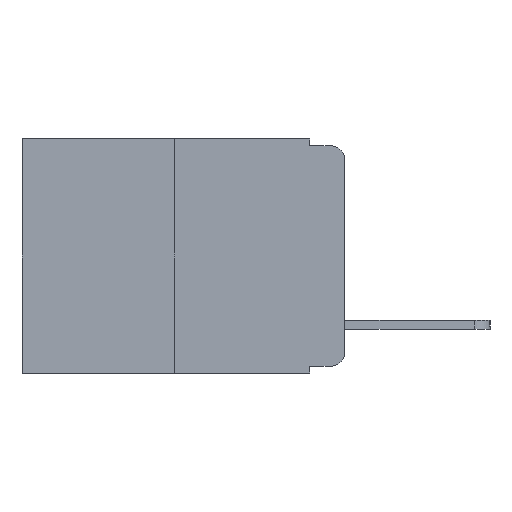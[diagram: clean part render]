
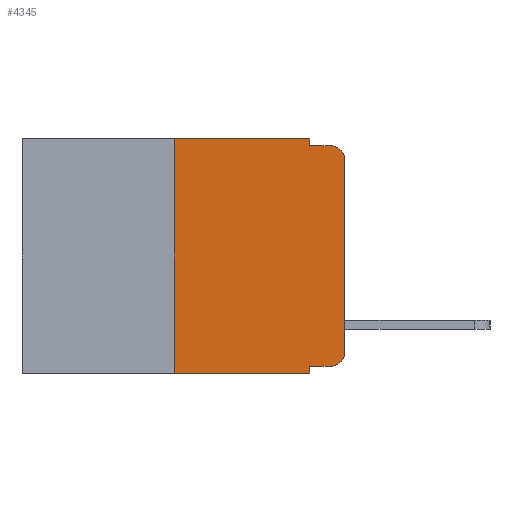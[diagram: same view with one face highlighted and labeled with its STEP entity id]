
A CAD part, left-side view. The second image highlights one B-rep face of the part: STEP entity #4345.
In plain terms, the highlighted planar face has unit normal (-1, 0, 0).
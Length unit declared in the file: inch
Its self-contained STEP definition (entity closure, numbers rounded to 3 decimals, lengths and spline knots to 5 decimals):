
#116 = VECTOR ( 'NONE', #1831, 39.37008 ) ;
#326 = CARTESIAN_POINT ( 'NONE',  ( 0., 0.051, -0.01 ) ) ;
#350 = CARTESIAN_POINT ( 'NONE',  ( 0., 0.02, -0.333 ) ) ;
#573 = VECTOR ( 'NONE', #5670, 39.37008 ) ;
#864 = CARTESIAN_POINT ( 'NONE',  ( 0., 0.473, 0. ) ) ;
#995 = EDGE_CURVE ( 'NONE', #1501, #5883, #3281, .T. ) ;
#1110 = DIRECTION ( 'NONE',  ( 0., -1., 0. ) ) ;
#1421 = VECTOR ( 'NONE', #14929, 39.37008 ) ;
#1501 = VERTEX_POINT ( 'NONE', #6995 ) ;
#1635 = ORIENTED_EDGE ( 'NONE', *, *, #4599, .F. ) ;
#1831 = DIRECTION ( 'NONE',  ( 0., 0., -1. ) ) ;
#1988 = CARTESIAN_POINT ( 'NONE',  ( 0., 0.25, 0. ) ) ;
#2081 = VERTEX_POINT ( 'NONE', #3625 ) ;
#2316 = CARTESIAN_POINT ( 'NONE',  ( 0., 0., -0.03 ) ) ;
#2392 = ORIENTED_EDGE ( 'NONE', *, *, #6445, .T. ) ;
#2616 = EDGE_CURVE ( 'NONE', #2081, #14643, #9075, .T. ) ;
#2891 = VERTEX_POINT ( 'NONE', #350 ) ;
#3139 = VECTOR ( 'NONE', #1110, 39.37008 ) ;
#3272 = LINE ( 'NONE', #5711, #3139 ) ;
#3277 = ORIENTED_EDGE ( 'NONE', *, *, #10185, .T. ) ;
#3281 = LINE ( 'NONE', #8940, #116 ) ;
#3625 = CARTESIAN_POINT ( 'NONE',  ( 0., 0.25, -0.343 ) ) ;
#3652 = AXIS2_PLACEMENT_3D ( 'NONE', #864, #13709, #5677 ) ;
#3986 = LINE ( 'NONE', #4136, #4137 ) ;
#4032 = AXIS2_PLACEMENT_3D ( 'NONE', #4738, #6208, #10890 ) ;
#4136 = CARTESIAN_POINT ( 'NONE',  ( 0., 0., 0. ) ) ;
#4137 = VECTOR ( 'NONE', #8644, 39.37008 ) ;
#4330 = ORIENTED_EDGE ( 'NONE', *, *, #12147, .T. ) ;
#4345 = ADVANCED_FACE ( 'NONE', ( #10354 ), #8130, .F. ) ;
#4388 = VERTEX_POINT ( 'NONE', #2316 ) ;
#4534 = VERTEX_POINT ( 'NONE', #11908 ) ;
#4599 = EDGE_CURVE ( 'NONE', #5883, #5077, #11755, .T. ) ;
#4738 = CARTESIAN_POINT ( 'NONE',  ( 0., 0.02, -0.313 ) ) ;
#4932 = CARTESIAN_POINT ( 'NONE',  ( 0., 0.02, -0.03 ) ) ;
#5077 = VERTEX_POINT ( 'NONE', #9718 ) ;
#5256 = CARTESIAN_POINT ( 'NONE',  ( 0., 0.473, 0. ) ) ;
#5670 = DIRECTION ( 'NONE',  ( 0., -1., 0. ) ) ;
#5677 = DIRECTION ( 'NONE',  ( 0., 0., -1. ) ) ;
#5711 = CARTESIAN_POINT ( 'NONE',  ( 0., 0.473, -0.343 ) ) ;
#5883 = VERTEX_POINT ( 'NONE', #6004 ) ;
#5895 = CARTESIAN_POINT ( 'NONE',  ( 0., 0.051, -0.333 ) ) ;
#5909 = CARTESIAN_POINT ( 'NONE',  ( 0., 0.051, -0.343 ) ) ;
#6004 = CARTESIAN_POINT ( 'NONE',  ( 0., 0.051, -0.01 ) ) ;
#6208 = DIRECTION ( 'NONE',  ( -1., 0., 0. ) ) ;
#6445 = EDGE_CURVE ( 'NONE', #4534, #4388, #3986, .T. ) ;
#6995 = CARTESIAN_POINT ( 'NONE',  ( 0., 0.051, 0. ) ) ;
#7309 = DIRECTION ( 'NONE',  ( -1., 0., 0. ) ) ;
#7410 = DIRECTION ( 'NONE',  ( 0., -1., 0. ) ) ;
#7966 = EDGE_LOOP ( 'NONE', ( #2392, #4330, #1635, #10959, #11152, #10036, #12329, #13815, #12493, #3277 ) ) ;
#8130 = PLANE ( 'NONE',  #3652 ) ;
#8278 = DIRECTION ( 'NONE',  ( 0., -1., 0. ) ) ;
#8307 = DIRECTION ( 'NONE',  ( 0., 0., -1. ) ) ;
#8644 = DIRECTION ( 'NONE',  ( 0., 0., 1. ) ) ;
#8940 = CARTESIAN_POINT ( 'NONE',  ( 0., 0.051, 0. ) ) ;
#9075 = LINE ( 'NONE', #14852, #1421 ) ;
#9117 = LINE ( 'NONE', #9195, #573 ) ;
#9195 = CARTESIAN_POINT ( 'NONE',  ( 0., 0.051, -0.333 ) ) ;
#9718 = CARTESIAN_POINT ( 'NONE',  ( 0., 0.02, -0.01 ) ) ;
#10036 = ORIENTED_EDGE ( 'NONE', *, *, #2616, .F. ) ;
#10185 = EDGE_CURVE ( 'NONE', #2891, #4534, #11129, .T. ) ;
#10354 = FACE_OUTER_BOUND ( 'NONE', #7966, .T. ) ;
#10542 = DIRECTION ( 'NONE',  ( 0., 0., -1. ) ) ;
#10698 = CARTESIAN_POINT ( 'NONE',  ( 0., 0.051, 0. ) ) ;
#10890 = DIRECTION ( 'NONE',  ( 0., 0., -1. ) ) ;
#10959 = ORIENTED_EDGE ( 'NONE', *, *, #995, .F. ) ;
#11019 = VECTOR ( 'NONE', #8278, 39.37008 ) ;
#11129 = CIRCLE ( 'NONE', #4032, 0.02 ) ;
#11152 = ORIENTED_EDGE ( 'NONE', *, *, #14902, .F. ) ;
#11278 = AXIS2_PLACEMENT_3D ( 'NONE', #4932, #7309, #8307 ) ;
#11522 = CIRCLE ( 'NONE', #11278, 0.02 ) ;
#11755 = LINE ( 'NONE', #326, #11019 ) ;
#11837 = EDGE_CURVE ( 'NONE', #14362, #2891, #9117, .T. ) ;
#11862 = LINE ( 'NONE', #10698, #14957 ) ;
#11908 = CARTESIAN_POINT ( 'NONE',  ( 0., 0., -0.313 ) ) ;
#12072 = EDGE_CURVE ( 'NONE', #2081, #12620, #3272, .T. ) ;
#12134 = EDGE_CURVE ( 'NONE', #14362, #12620, #11862, .T. ) ;
#12147 = EDGE_CURVE ( 'NONE', #4388, #5077, #11522, .T. ) ;
#12329 = ORIENTED_EDGE ( 'NONE', *, *, #12072, .T. ) ;
#12348 = LINE ( 'NONE', #5256, #12349 ) ;
#12349 = VECTOR ( 'NONE', #7410, 39.37008 ) ;
#12493 = ORIENTED_EDGE ( 'NONE', *, *, #11837, .T. ) ;
#12620 = VERTEX_POINT ( 'NONE', #5909 ) ;
#13709 = DIRECTION ( 'NONE',  ( 1., 0., 0. ) ) ;
#13815 = ORIENTED_EDGE ( 'NONE', *, *, #12134, .F. ) ;
#14362 = VERTEX_POINT ( 'NONE', #5895 ) ;
#14643 = VERTEX_POINT ( 'NONE', #1988 ) ;
#14852 = CARTESIAN_POINT ( 'NONE',  ( 0., 0.25, 0. ) ) ;
#14902 = EDGE_CURVE ( 'NONE', #14643, #1501, #12348, .T. ) ;
#14929 = DIRECTION ( 'NONE',  ( 0., 0., 1. ) ) ;
#14957 = VECTOR ( 'NONE', #10542, 39.37008 ) ;
